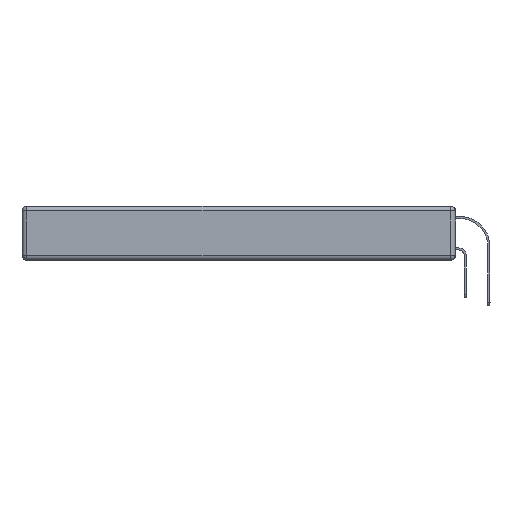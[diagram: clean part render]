
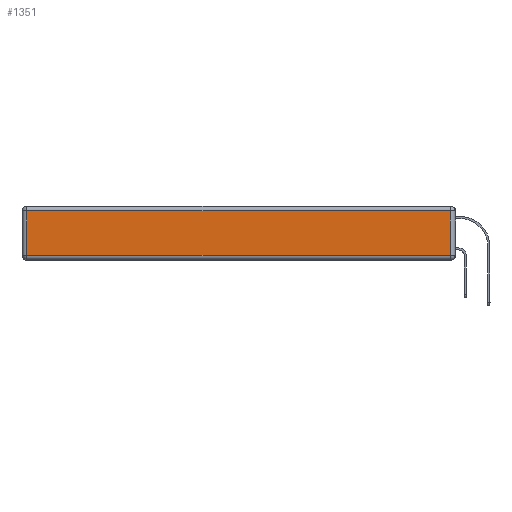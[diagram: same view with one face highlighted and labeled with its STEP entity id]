
A CAD part, left-side view. The second image highlights one B-rep face of the part: STEP entity #1351.
In plain terms, the highlighted planar face has unit normal (-1, 0, 0).
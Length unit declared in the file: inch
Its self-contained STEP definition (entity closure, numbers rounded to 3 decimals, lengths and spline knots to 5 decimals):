
#167 = VERTEX_POINT ( 'NONE', #2140 ) ;
#343 = CARTESIAN_POINT ( 'NONE',  ( 0., 2.72, -0.313 ) ) ;
#1300 = ORIENTED_EDGE ( 'NONE', *, *, #1921, .T. ) ;
#1351 = ADVANCED_FACE ( 'NONE', ( #3076 ), #14738, .T. ) ;
#1921 = EDGE_CURVE ( 'NONE', #2259, #14729, #18144, .T. ) ;
#2140 = CARTESIAN_POINT ( 'NONE',  ( 0., 0.03, -0.313 ) ) ;
#2259 = VERTEX_POINT ( 'NONE', #5582 ) ;
#2577 = LINE ( 'NONE', #6005, #4934 ) ;
#2677 = ORIENTED_EDGE ( 'NONE', *, *, #8813, .T. ) ;
#3076 = FACE_OUTER_BOUND ( 'NONE', #9737, .T. ) ;
#3261 = DIRECTION ( 'NONE',  ( 0., 0., 1. ) ) ;
#3695 = VECTOR ( 'NONE', #13741, 39.37008 ) ;
#4357 = DIRECTION ( 'NONE',  ( 0., -1., 0. ) ) ;
#4934 = VECTOR ( 'NONE', #4357, 39.37008 ) ;
#5582 = CARTESIAN_POINT ( 'NONE',  ( 0., 0.03, -0.03 ) ) ;
#6005 = CARTESIAN_POINT ( 'NONE',  ( 0., 0., -0.313 ) ) ;
#6143 = VECTOR ( 'NONE', #13938, 39.37008 ) ;
#6392 = ORIENTED_EDGE ( 'NONE', *, *, #7623, .T. ) ;
#7272 = CARTESIAN_POINT ( 'NONE',  ( 0., 0., -0.343 ) ) ;
#7623 = EDGE_CURVE ( 'NONE', #14729, #8437, #15782, .T. ) ;
#8149 = CARTESIAN_POINT ( 'NONE',  ( 0., 2.72, -0.343 ) ) ;
#8437 = VERTEX_POINT ( 'NONE', #343 ) ;
#8813 = EDGE_CURVE ( 'NONE', #167, #2259, #10620, .T. ) ;
#9419 = CARTESIAN_POINT ( 'NONE',  ( 0., 2.75, -0.03 ) ) ;
#9737 = EDGE_LOOP ( 'NONE', ( #14067, #2677, #1300, #6392 ) ) ;
#10620 = LINE ( 'NONE', #16774, #15582 ) ;
#12603 = CARTESIAN_POINT ( 'NONE',  ( 0., 2.72, -0.03 ) ) ;
#13741 = DIRECTION ( 'NONE',  ( 0., 1., 0. ) ) ;
#13938 = DIRECTION ( 'NONE',  ( 0., 0., -1. ) ) ;
#14067 = ORIENTED_EDGE ( 'NONE', *, *, #16660, .T. ) ;
#14729 = VERTEX_POINT ( 'NONE', #12603 ) ;
#14738 = PLANE ( 'NONE',  #16293 ) ;
#15029 = DIRECTION ( 'NONE',  ( 0., 0., 1. ) ) ;
#15582 = VECTOR ( 'NONE', #3261, 39.37008 ) ;
#15782 = LINE ( 'NONE', #8149, #6143 ) ;
#16293 = AXIS2_PLACEMENT_3D ( 'NONE', #7272, #16396, #15029 ) ;
#16396 = DIRECTION ( 'NONE',  ( -1., 0., 0. ) ) ;
#16660 = EDGE_CURVE ( 'NONE', #8437, #167, #2577, .T. ) ;
#16774 = CARTESIAN_POINT ( 'NONE',  ( 0., 0.03, -0.343 ) ) ;
#18144 = LINE ( 'NONE', #9419, #3695 ) ;
